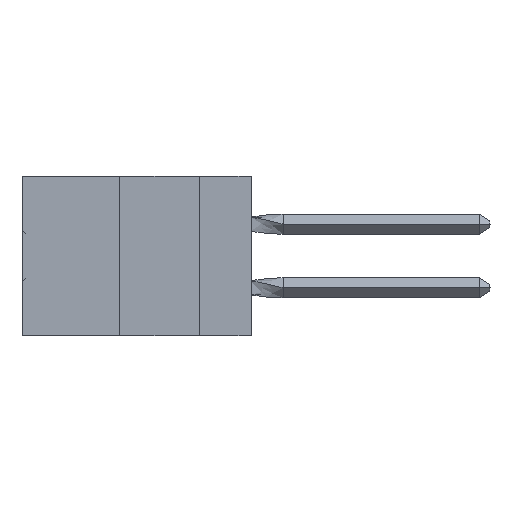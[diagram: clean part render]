
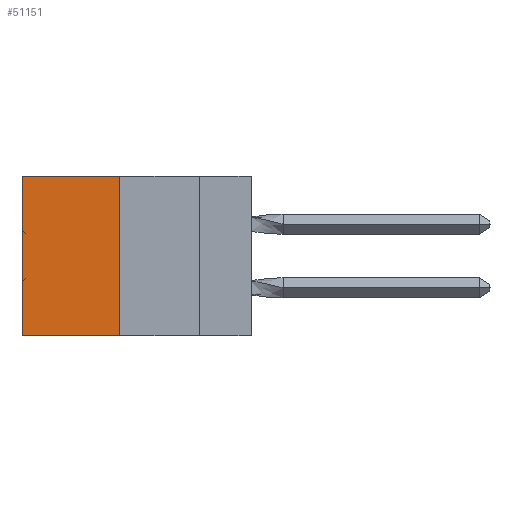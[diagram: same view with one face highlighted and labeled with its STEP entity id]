
A CAD part, left-side view. The second image highlights one B-rep face of the part: STEP entity #51151.
In plain terms, the highlighted planar face has unit normal (-1, 0, 0).
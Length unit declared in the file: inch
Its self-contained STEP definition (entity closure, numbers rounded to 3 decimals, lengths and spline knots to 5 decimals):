
#2287 = LINE ( 'NONE', #12869, #43920 ) ;
#2780 = AXIS2_PLACEMENT_3D ( 'NONE', #35497, #22059, #30562 ) ;
#8338 = VERTEX_POINT ( 'NONE', #31366 ) ;
#8507 = LINE ( 'NONE', #53311, #48780 ) ;
#10260 = ORIENTED_EDGE ( 'NONE', *, *, #38884, .T. ) ;
#12869 = CARTESIAN_POINT ( 'NONE',  ( 0.305, 0.413, 0. ) ) ;
#13297 = VECTOR ( 'NONE', #23964, 39.37008 ) ;
#16271 = CARTESIAN_POINT ( 'NONE',  ( 0.305, 0.413, -0.5 ) ) ;
#17558 = EDGE_CURVE ( 'NONE', #8338, #36678, #41474, .T. ) ;
#18178 = VERTEX_POINT ( 'NONE', #37109 ) ;
#21441 = ORIENTED_EDGE ( 'NONE', *, *, #17558, .F. ) ;
#22059 = DIRECTION ( 'NONE',  ( 1., 0., 0. ) ) ;
#22145 = DIRECTION ( 'NONE',  ( 0., 0., -1. ) ) ;
#22248 = CARTESIAN_POINT ( 'NONE',  ( 0.305, 0.72, -0.5 ) ) ;
#22906 = DIRECTION ( 'NONE',  ( 0., 1., 0. ) ) ;
#23964 = DIRECTION ( 'NONE',  ( 0., 0., -1. ) ) ;
#24277 = ORIENTED_EDGE ( 'NONE', *, *, #26080, .T. ) ;
#26080 = EDGE_CURVE ( 'NONE', #18178, #36678, #8507, .T. ) ;
#29092 = EDGE_LOOP ( 'NONE', ( #24277, #21441, #37599, #10260 ) ) ;
#29224 = VERTEX_POINT ( 'NONE', #32624 ) ;
#30562 = DIRECTION ( 'NONE',  ( 0., 0., -1. ) ) ;
#31366 = CARTESIAN_POINT ( 'NONE',  ( 0.305, 0.413, -0.5 ) ) ;
#31449 = FACE_OUTER_BOUND ( 'NONE', #29092, .T. ) ;
#32624 = CARTESIAN_POINT ( 'NONE',  ( 0.305, 0.413, 0. ) ) ;
#34323 = EDGE_CURVE ( 'NONE', #29224, #8338, #38703, .T. ) ;
#35497 = CARTESIAN_POINT ( 'NONE',  ( 0.305, 0.413, -0.5 ) ) ;
#36678 = VERTEX_POINT ( 'NONE', #22248 ) ;
#37109 = CARTESIAN_POINT ( 'NONE',  ( 0.305, 0.72, 0. ) ) ;
#37599 = ORIENTED_EDGE ( 'NONE', *, *, #34323, .F. ) ;
#37908 = VECTOR ( 'NONE', #38758, 39.37008 ) ;
#38703 = LINE ( 'NONE', #54759, #13297 ) ;
#38758 = DIRECTION ( 'NONE',  ( 0., 1., 0. ) ) ;
#38884 = EDGE_CURVE ( 'NONE', #29224, #18178, #2287, .T. ) ;
#41474 = LINE ( 'NONE', #16271, #37908 ) ;
#43920 = VECTOR ( 'NONE', #22906, 39.37008 ) ;
#48780 = VECTOR ( 'NONE', #22145, 39.37008 ) ;
#49109 = PLANE ( 'NONE',  #2780 ) ;
#51151 = ADVANCED_FACE ( 'NONE', ( #31449 ), #49109, .F. ) ;
#53311 = CARTESIAN_POINT ( 'NONE',  ( 0.305, 0.72, -0.5 ) ) ;
#54759 = CARTESIAN_POINT ( 'NONE',  ( 0.305, 0.413, -0.5 ) ) ;
